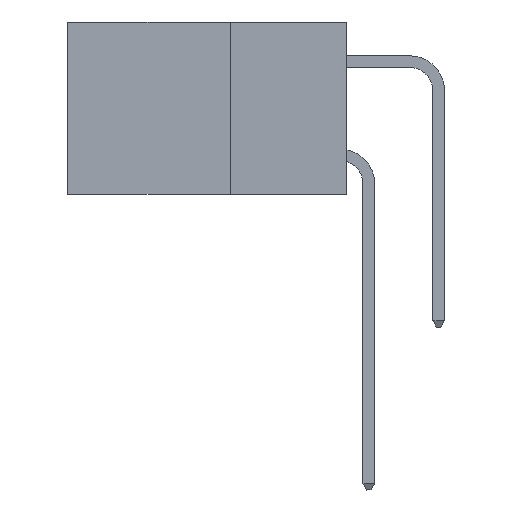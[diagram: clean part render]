
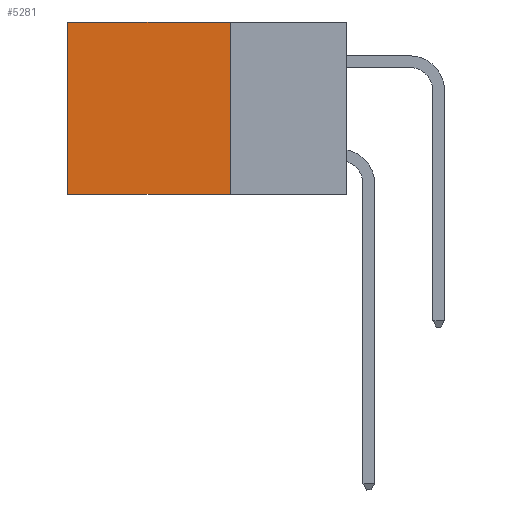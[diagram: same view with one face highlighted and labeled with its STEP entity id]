
A CAD part, left-side view. The second image highlights one B-rep face of the part: STEP entity #5281.
In plain terms, the highlighted planar face has unit normal (-1, 0, 0).
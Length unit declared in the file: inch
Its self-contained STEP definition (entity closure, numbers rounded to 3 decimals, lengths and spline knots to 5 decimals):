
#741 = DIRECTION ( 'NONE',  ( 0., 0., -1. ) ) ;
#913 = DIRECTION ( 'NONE',  ( 0., 0., -1. ) ) ;
#1063 = CARTESIAN_POINT ( 'NONE',  ( 0.2875, 0.6, 0. ) ) ;
#1526 = LINE ( 'NONE', #1661, #14443 ) ;
#1661 = CARTESIAN_POINT ( 'NONE',  ( 0.2875, 0.25, -0.37 ) ) ;
#1790 = CARTESIAN_POINT ( 'NONE',  ( 0.2875, 0.25, -0.37 ) ) ;
#2195 = CARTESIAN_POINT ( 'NONE',  ( 0.2875, 0.6, 0. ) ) ;
#3651 = LINE ( 'NONE', #1063, #5519 ) ;
#4105 = VERTEX_POINT ( 'NONE', #2195 ) ;
#4314 = VECTOR ( 'NONE', #20103, 39.37008 ) ;
#4992 = EDGE_CURVE ( 'NONE', #4105, #23188, #3651, .T. ) ;
#5281 = ADVANCED_FACE ( 'NONE', ( #20525 ), #24284, .F. ) ;
#5519 = VECTOR ( 'NONE', #913, 39.37008 ) ;
#6216 = CARTESIAN_POINT ( 'NONE',  ( 0.2875, 0.25, 0. ) ) ;
#7392 = LINE ( 'NONE', #9279, #4314 ) ;
#9269 = CARTESIAN_POINT ( 'NONE',  ( 0.2875, 0.6, -0.37 ) ) ;
#9279 = CARTESIAN_POINT ( 'NONE',  ( 0.2875, 0.25, 0. ) ) ;
#9418 = CARTESIAN_POINT ( 'NONE',  ( 0.2875, 0.25, 0. ) ) ;
#10350 = DIRECTION ( 'NONE',  ( 0., 1., 0. ) ) ;
#11704 = EDGE_CURVE ( 'NONE', #15580, #23188, #1526, .T. ) ;
#12599 = VERTEX_POINT ( 'NONE', #6216 ) ;
#13802 = ORIENTED_EDGE ( 'NONE', *, *, #4992, .T. ) ;
#14374 = EDGE_CURVE ( 'NONE', #12599, #4105, #7392, .T. ) ;
#14412 = EDGE_CURVE ( 'NONE', #12599, #15580, #18379, .T. ) ;
#14443 = VECTOR ( 'NONE', #10350, 39.37008 ) ;
#15580 = VERTEX_POINT ( 'NONE', #1790 ) ;
#16468 = ORIENTED_EDGE ( 'NONE', *, *, #11704, .F. ) ;
#18379 = LINE ( 'NONE', #27221, #25066 ) ;
#18473 = AXIS2_PLACEMENT_3D ( 'NONE', #9418, #24867, #741 ) ;
#19385 = EDGE_LOOP ( 'NONE', ( #13802, #16468, #26976, #26209 ) ) ;
#20103 = DIRECTION ( 'NONE',  ( 0., 1., 0. ) ) ;
#20525 = FACE_OUTER_BOUND ( 'NONE', #19385, .T. ) ;
#22687 = DIRECTION ( 'NONE',  ( 0., 0., -1. ) ) ;
#23188 = VERTEX_POINT ( 'NONE', #9269 ) ;
#24284 = PLANE ( 'NONE',  #18473 ) ;
#24867 = DIRECTION ( 'NONE',  ( 1., 0., 0. ) ) ;
#25066 = VECTOR ( 'NONE', #22687, 39.37008 ) ;
#26209 = ORIENTED_EDGE ( 'NONE', *, *, #14374, .T. ) ;
#26976 = ORIENTED_EDGE ( 'NONE', *, *, #14412, .F. ) ;
#27221 = CARTESIAN_POINT ( 'NONE',  ( 0.2875, 0.25, 0. ) ) ;
